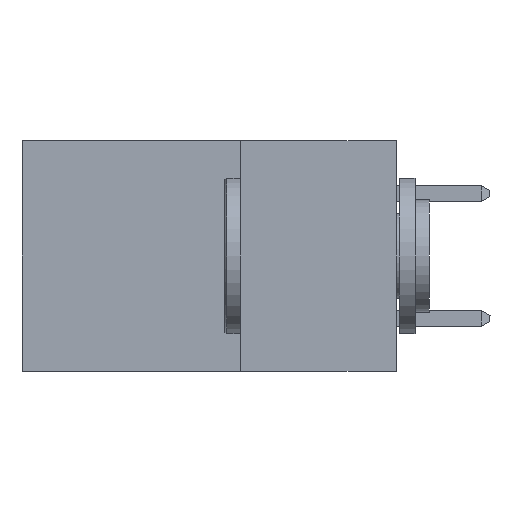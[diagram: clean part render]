
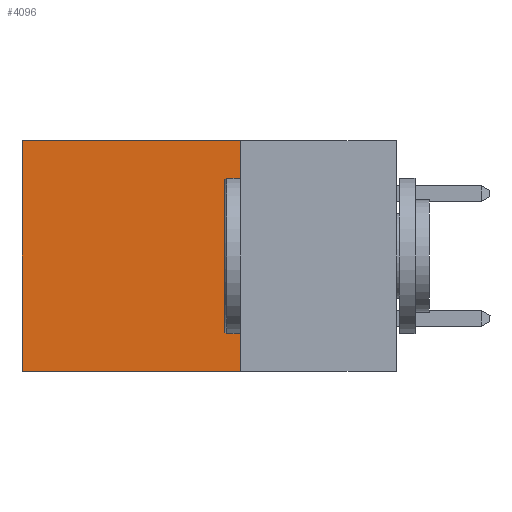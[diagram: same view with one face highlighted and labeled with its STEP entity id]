
A CAD part, left-side view. The second image highlights one B-rep face of the part: STEP entity #4096.
In plain terms, the highlighted planar face has unit normal (-1, 0, 0).
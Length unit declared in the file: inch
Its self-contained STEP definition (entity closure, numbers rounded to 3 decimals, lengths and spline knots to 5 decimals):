
#294 = VECTOR ( 'NONE', #11853, 39.37008 ) ;
#949 = CARTESIAN_POINT ( 'NONE',  ( 0.298, 0.25, 0. ) ) ;
#1005 = DIRECTION ( 'NONE',  ( 0., 1., 0. ) ) ;
#1034 = DIRECTION ( 'NONE',  ( 0., 0., -1. ) ) ;
#2038 = CARTESIAN_POINT ( 'NONE',  ( 0.298, 0.25, 0. ) ) ;
#2363 = VERTEX_POINT ( 'NONE', #4403 ) ;
#2431 = VECTOR ( 'NONE', #19001, 39.37008 ) ;
#2997 = VECTOR ( 'NONE', #1005, 39.37008 ) ;
#3469 = EDGE_CURVE ( 'NONE', #18040, #18118, #16231, .T. ) ;
#3670 = CARTESIAN_POINT ( 'NONE',  ( 0.298, 0.6, 0. ) ) ;
#4082 = EDGE_LOOP ( 'NONE', ( #10621, #12529, #23555, #7795 ) ) ;
#4096 = ADVANCED_FACE ( 'NONE', ( #23402 ), #10410, .F. ) ;
#4103 = VERTEX_POINT ( 'NONE', #17229 ) ;
#4403 = CARTESIAN_POINT ( 'NONE',  ( 0.298, 0.25, -0.37 ) ) ;
#5001 = CARTESIAN_POINT ( 'NONE',  ( 0.298, 0.25, -0.37 ) ) ;
#7795 = ORIENTED_EDGE ( 'NONE', *, *, #3469, .T. ) ;
#9374 = DIRECTION ( 'NONE',  ( 1., 0., 0. ) ) ;
#9460 = DIRECTION ( 'NONE',  ( 0., 0., -1. ) ) ;
#9641 = LINE ( 'NONE', #5001, #2997 ) ;
#10410 = PLANE ( 'NONE',  #15794 ) ;
#10621 = ORIENTED_EDGE ( 'NONE', *, *, #19827, .T. ) ;
#10843 = CARTESIAN_POINT ( 'NONE',  ( 0.298, 0.6, 0. ) ) ;
#11392 = CARTESIAN_POINT ( 'NONE',  ( 0.298, 0.25, 0. ) ) ;
#11840 = VECTOR ( 'NONE', #1034, 39.37008 ) ;
#11853 = DIRECTION ( 'NONE',  ( 0., 1., 0. ) ) ;
#12529 = ORIENTED_EDGE ( 'NONE', *, *, #21002, .F. ) ;
#13070 = EDGE_CURVE ( 'NONE', #18040, #2363, #22628, .T. ) ;
#15677 = LINE ( 'NONE', #3670, #2431 ) ;
#15794 = AXIS2_PLACEMENT_3D ( 'NONE', #24262, #9374, #9460 ) ;
#16231 = LINE ( 'NONE', #2038, #294 ) ;
#17229 = CARTESIAN_POINT ( 'NONE',  ( 0.298, 0.6, -0.37 ) ) ;
#18040 = VERTEX_POINT ( 'NONE', #11392 ) ;
#18118 = VERTEX_POINT ( 'NONE', #10843 ) ;
#19001 = DIRECTION ( 'NONE',  ( 0., 0., -1. ) ) ;
#19827 = EDGE_CURVE ( 'NONE', #18118, #4103, #15677, .T. ) ;
#21002 = EDGE_CURVE ( 'NONE', #2363, #4103, #9641, .T. ) ;
#22628 = LINE ( 'NONE', #949, #11840 ) ;
#23402 = FACE_OUTER_BOUND ( 'NONE', #4082, .T. ) ;
#23555 = ORIENTED_EDGE ( 'NONE', *, *, #13070, .F. ) ;
#24262 = CARTESIAN_POINT ( 'NONE',  ( 0.298, 0.25, 0. ) ) ;
